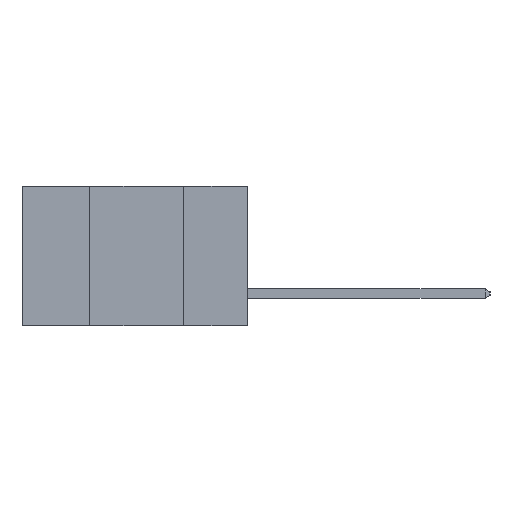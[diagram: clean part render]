
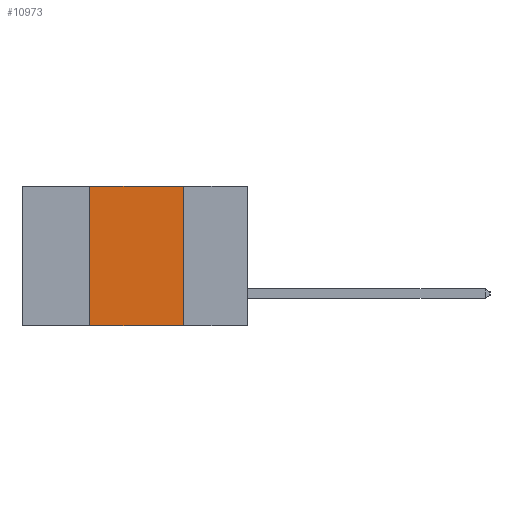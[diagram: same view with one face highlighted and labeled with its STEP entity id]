
A CAD part, left-side view. The second image highlights one B-rep face of the part: STEP entity #10973.
In plain terms, the highlighted planar face has unit normal (-1, 0, 0).
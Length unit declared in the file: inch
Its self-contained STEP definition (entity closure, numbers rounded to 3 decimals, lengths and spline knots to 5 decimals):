
#231 = VERTEX_POINT ( 'NONE', #3785 ) ;
#516 = ORIENTED_EDGE ( 'NONE', *, *, #1328, .F. ) ;
#939 = CARTESIAN_POINT ( 'NONE',  ( 0., 0.17, 0. ) ) ;
#1011 = VERTEX_POINT ( 'NONE', #3870 ) ;
#1147 = EDGE_LOOP ( 'NONE', ( #11343, #516, #1212, #2466 ) ) ;
#1212 = ORIENTED_EDGE ( 'NONE', *, *, #14504, .F. ) ;
#1328 = EDGE_CURVE ( 'NONE', #231, #9294, #1401, .T. ) ;
#1401 = LINE ( 'NONE', #3067, #16758 ) ;
#2466 = ORIENTED_EDGE ( 'NONE', *, *, #13270, .T. ) ;
#3067 = CARTESIAN_POINT ( 'NONE',  ( 0., 0.6, 0. ) ) ;
#3785 = CARTESIAN_POINT ( 'NONE',  ( 0., 0.42, 0. ) ) ;
#3870 = CARTESIAN_POINT ( 'NONE',  ( 0., 0.17, -0.37 ) ) ;
#4426 = VECTOR ( 'NONE', #11692, 39.37008 ) ;
#4573 = DIRECTION ( 'NONE',  ( 0., -1., 0. ) ) ;
#5330 = DIRECTION ( 'NONE',  ( 1., 0., 0. ) ) ;
#5334 = LINE ( 'NONE', #21116, #14932 ) ;
#6287 = LINE ( 'NONE', #20884, #4426 ) ;
#8117 = DIRECTION ( 'NONE',  ( 0., 0., -1. ) ) ;
#9076 = CARTESIAN_POINT ( 'NONE',  ( 0., 0.6, 0. ) ) ;
#9294 = VERTEX_POINT ( 'NONE', #939 ) ;
#10519 = VECTOR ( 'NONE', #20854, 39.37008 ) ;
#10973 = ADVANCED_FACE ( 'NONE', ( #15127 ), #11124, .F. ) ;
#11124 = PLANE ( 'NONE',  #16258 ) ;
#11343 = ORIENTED_EDGE ( 'NONE', *, *, #15731, .F. ) ;
#11692 = DIRECTION ( 'NONE',  ( 0., -1., 0. ) ) ;
#13270 = EDGE_CURVE ( 'NONE', #19148, #1011, #6287, .T. ) ;
#14504 = EDGE_CURVE ( 'NONE', #19148, #231, #20395, .T. ) ;
#14795 = CARTESIAN_POINT ( 'NONE',  ( 0., 0.42, -0.37 ) ) ;
#14932 = VECTOR ( 'NONE', #8117, 39.37008 ) ;
#15127 = FACE_OUTER_BOUND ( 'NONE', #1147, .T. ) ;
#15258 = CARTESIAN_POINT ( 'NONE',  ( 0., 0.42, 0. ) ) ;
#15731 = EDGE_CURVE ( 'NONE', #9294, #1011, #5334, .T. ) ;
#16258 = AXIS2_PLACEMENT_3D ( 'NONE', #9076, #5330, #18549 ) ;
#16758 = VECTOR ( 'NONE', #4573, 39.37008 ) ;
#18549 = DIRECTION ( 'NONE',  ( 0., 0., -1. ) ) ;
#19148 = VERTEX_POINT ( 'NONE', #14795 ) ;
#20395 = LINE ( 'NONE', #15258, #10519 ) ;
#20854 = DIRECTION ( 'NONE',  ( 0., 0., 1. ) ) ;
#20884 = CARTESIAN_POINT ( 'NONE',  ( 0., 0.6, -0.37 ) ) ;
#21116 = CARTESIAN_POINT ( 'NONE',  ( 0., 0.17, 0. ) ) ;
